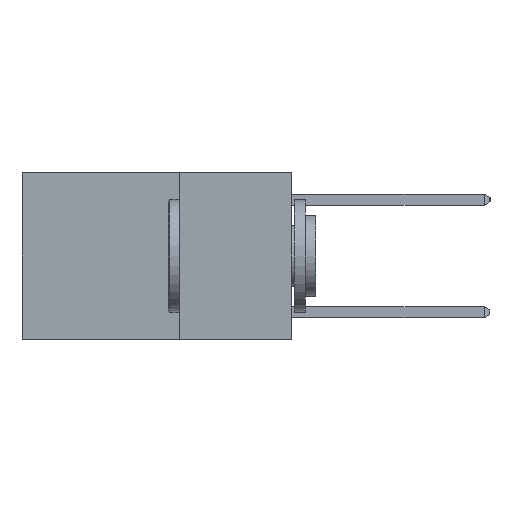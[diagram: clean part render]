
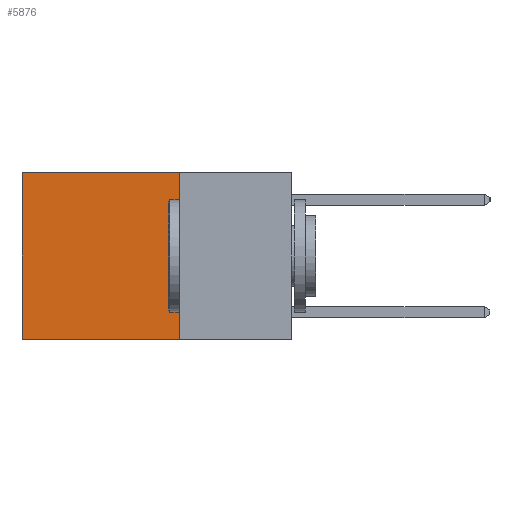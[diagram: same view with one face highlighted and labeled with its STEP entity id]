
A CAD part, left-side view. The second image highlights one B-rep face of the part: STEP entity #5876.
In plain terms, the highlighted planar face has unit normal (-1, 0, 0).
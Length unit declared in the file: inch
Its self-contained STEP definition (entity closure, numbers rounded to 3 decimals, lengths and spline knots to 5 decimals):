
#236 = ORIENTED_EDGE ( 'NONE', *, *, #3976, .T. ) ;
#365 = ORIENTED_EDGE ( 'NONE', *, *, #1387, .F. ) ;
#419 = EDGE_CURVE ( 'NONE', #1751, #7878, #10670, .T. ) ;
#1387 = EDGE_CURVE ( 'NONE', #3681, #7878, #9619, .T. ) ;
#1629 = EDGE_LOOP ( 'NONE', ( #10231, #365, #9087, #236 ) ) ;
#1751 = VERTEX_POINT ( 'NONE', #7324 ) ;
#1794 = CARTESIAN_POINT ( 'NONE',  ( 0.2625, 0.25, 0. ) ) ;
#2375 = LINE ( 'NONE', #1794, #8951 ) ;
#2694 = DIRECTION ( 'NONE',  ( 0., 0., -1. ) ) ;
#2707 = CARTESIAN_POINT ( 'NONE',  ( 0.2625, 0.25, 0. ) ) ;
#2753 = DIRECTION ( 'NONE',  ( 0., 1., 0. ) ) ;
#2842 = CARTESIAN_POINT ( 'NONE',  ( 0.2625, 0.25, 0. ) ) ;
#3114 = CARTESIAN_POINT ( 'NONE',  ( 0.2625, 0.25, 0. ) ) ;
#3145 = CARTESIAN_POINT ( 'NONE',  ( 0.2625, 0.6, -0.37 ) ) ;
#3475 = VECTOR ( 'NONE', #10217, 39.37008 ) ;
#3681 = VERTEX_POINT ( 'NONE', #5073 ) ;
#3976 = EDGE_CURVE ( 'NONE', #7167, #1751, #8724, .T. ) ;
#4059 = DIRECTION ( 'NONE',  ( 1., 0., 0. ) ) ;
#5073 = CARTESIAN_POINT ( 'NONE',  ( 0.2625, 0.25, -0.37 ) ) ;
#5552 = EDGE_CURVE ( 'NONE', #7167, #3681, #2375, .T. ) ;
#5876 = ADVANCED_FACE ( 'NONE', ( #8808 ), #8488, .F. ) ;
#6736 = DIRECTION ( 'NONE',  ( 0., 1., 0. ) ) ;
#6873 = CARTESIAN_POINT ( 'NONE',  ( 0.2625, 0.25, -0.37 ) ) ;
#7167 = VERTEX_POINT ( 'NONE', #2842 ) ;
#7324 = CARTESIAN_POINT ( 'NONE',  ( 0.2625, 0.6, 0. ) ) ;
#7878 = VERTEX_POINT ( 'NONE', #3145 ) ;
#8488 = PLANE ( 'NONE',  #11512 ) ;
#8724 = LINE ( 'NONE', #2707, #10869 ) ;
#8808 = FACE_OUTER_BOUND ( 'NONE', #1629, .T. ) ;
#8935 = CARTESIAN_POINT ( 'NONE',  ( 0.2625, 0.6, 0. ) ) ;
#8951 = VECTOR ( 'NONE', #2694, 39.37008 ) ;
#9087 = ORIENTED_EDGE ( 'NONE', *, *, #5552, .F. ) ;
#9619 = LINE ( 'NONE', #6873, #11437 ) ;
#10217 = DIRECTION ( 'NONE',  ( 0., 0., -1. ) ) ;
#10231 = ORIENTED_EDGE ( 'NONE', *, *, #419, .T. ) ;
#10333 = DIRECTION ( 'NONE',  ( 0., 0., -1. ) ) ;
#10670 = LINE ( 'NONE', #8935, #3475 ) ;
#10869 = VECTOR ( 'NONE', #2753, 39.37008 ) ;
#11437 = VECTOR ( 'NONE', #6736, 39.37008 ) ;
#11512 = AXIS2_PLACEMENT_3D ( 'NONE', #3114, #4059, #10333 ) ;
